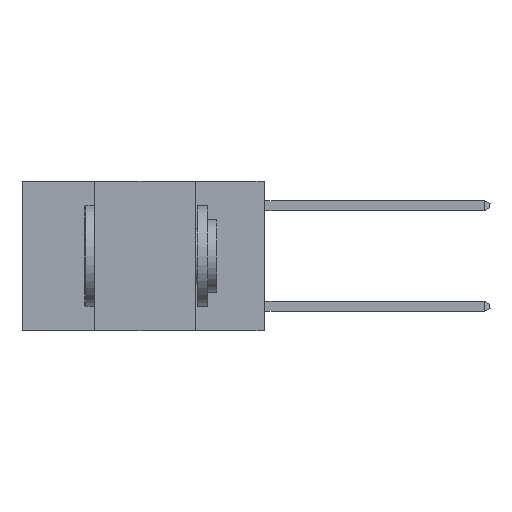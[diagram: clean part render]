
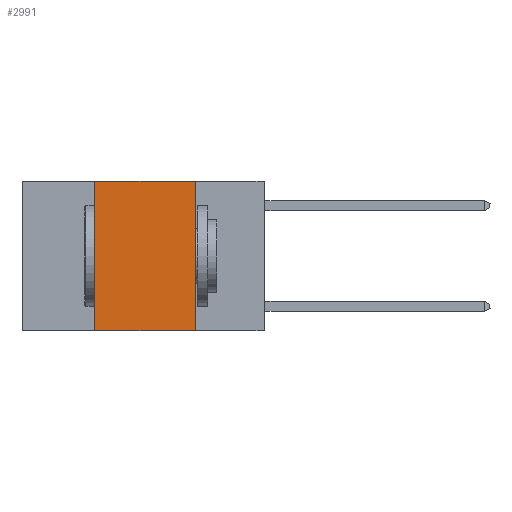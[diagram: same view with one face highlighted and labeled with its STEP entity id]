
A CAD part, left-side view. The second image highlights one B-rep face of the part: STEP entity #2991.
In plain terms, the highlighted planar face has unit normal (-1, 0, 0).
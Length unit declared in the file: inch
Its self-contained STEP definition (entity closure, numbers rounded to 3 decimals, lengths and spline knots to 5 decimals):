
#117 = CARTESIAN_POINT ( 'NONE',  ( 0., 0.42, 0. ) ) ;
#244 = VECTOR ( 'NONE', #12722, 39.37008 ) ;
#328 = EDGE_LOOP ( 'NONE', ( #1460, #15394, #16146, #6469 ) ) ;
#1071 = DIRECTION ( 'NONE',  ( 0., -1., 0. ) ) ;
#1460 = ORIENTED_EDGE ( 'NONE', *, *, #21586, .F. ) ;
#2051 = VECTOR ( 'NONE', #14703, 39.37008 ) ;
#2412 = DIRECTION ( 'NONE',  ( 0., 0., -1. ) ) ;
#2484 = LINE ( 'NONE', #7908, #2051 ) ;
#2645 = VERTEX_POINT ( 'NONE', #3205 ) ;
#2991 = ADVANCED_FACE ( 'NONE', ( #19407 ), #10873, .F. ) ;
#3006 = CARTESIAN_POINT ( 'NONE',  ( 0., 0.42, 0. ) ) ;
#3205 = CARTESIAN_POINT ( 'NONE',  ( 0., 0.42, -0.37 ) ) ;
#4758 = LINE ( 'NONE', #3006, #9990 ) ;
#5912 = LINE ( 'NONE', #15724, #244 ) ;
#6469 = ORIENTED_EDGE ( 'NONE', *, *, #9872, .T. ) ;
#7908 = CARTESIAN_POINT ( 'NONE',  ( 0., 0.17, 0. ) ) ;
#9088 = CARTESIAN_POINT ( 'NONE',  ( 0., 0.17, 0. ) ) ;
#9397 = EDGE_CURVE ( 'NONE', #13308, #17578, #19614, .T. ) ;
#9872 = EDGE_CURVE ( 'NONE', #2645, #20844, #5912, .T. ) ;
#9990 = VECTOR ( 'NONE', #13023, 39.37008 ) ;
#10873 = PLANE ( 'NONE',  #14325 ) ;
#10985 = CARTESIAN_POINT ( 'NONE',  ( 0., 0.6, 0. ) ) ;
#12722 = DIRECTION ( 'NONE',  ( 0., -1., 0. ) ) ;
#13023 = DIRECTION ( 'NONE',  ( 0., 0., 1. ) ) ;
#13308 = VERTEX_POINT ( 'NONE', #117 ) ;
#14325 = AXIS2_PLACEMENT_3D ( 'NONE', #10985, #17621, #2412 ) ;
#14520 = CARTESIAN_POINT ( 'NONE',  ( 0., 0.6, 0. ) ) ;
#14703 = DIRECTION ( 'NONE',  ( 0., 0., -1. ) ) ;
#15394 = ORIENTED_EDGE ( 'NONE', *, *, #9397, .F. ) ;
#15724 = CARTESIAN_POINT ( 'NONE',  ( 0., 0.6, -0.37 ) ) ;
#16146 = ORIENTED_EDGE ( 'NONE', *, *, #16770, .F. ) ;
#16770 = EDGE_CURVE ( 'NONE', #2645, #13308, #4758, .T. ) ;
#17578 = VERTEX_POINT ( 'NONE', #9088 ) ;
#17621 = DIRECTION ( 'NONE',  ( 1., 0., 0. ) ) ;
#18669 = VECTOR ( 'NONE', #1071, 39.37008 ) ;
#19407 = FACE_OUTER_BOUND ( 'NONE', #328, .T. ) ;
#19614 = LINE ( 'NONE', #14520, #18669 ) ;
#20835 = CARTESIAN_POINT ( 'NONE',  ( 0., 0.17, -0.37 ) ) ;
#20844 = VERTEX_POINT ( 'NONE', #20835 ) ;
#21586 = EDGE_CURVE ( 'NONE', #17578, #20844, #2484, .T. ) ;
